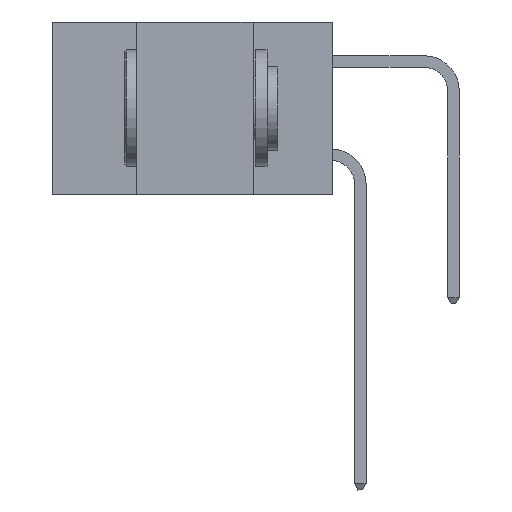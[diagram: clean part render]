
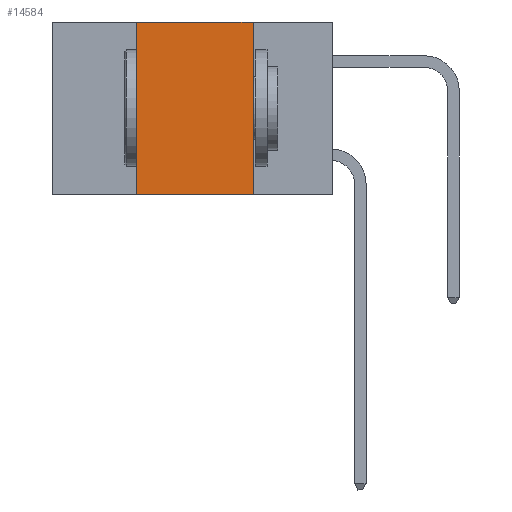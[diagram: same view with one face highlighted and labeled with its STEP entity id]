
A CAD part, left-side view. The second image highlights one B-rep face of the part: STEP entity #14584.
In plain terms, the highlighted planar face has unit normal (-1, 0, 0).
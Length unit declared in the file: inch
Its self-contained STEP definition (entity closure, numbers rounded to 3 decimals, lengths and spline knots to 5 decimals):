
#2361 = CARTESIAN_POINT ( 'NONE',  ( 0., 0.17, -0.37 ) ) ;
#2977 = CARTESIAN_POINT ( 'NONE',  ( 0., 0.6, 0. ) ) ;
#3004 = CARTESIAN_POINT ( 'NONE',  ( 0., 0.42, 0. ) ) ;
#4035 = CARTESIAN_POINT ( 'NONE',  ( 0., 0.42, -0.37 ) ) ;
#4650 = CARTESIAN_POINT ( 'NONE',  ( 0., 0.17, -0.37 ) ) ;
#4989 = AXIS2_PLACEMENT_3D ( 'NONE', #2977, #19009, #5336 ) ;
#5336 = DIRECTION ( 'NONE',  ( 0., 0., -1. ) ) ;
#6308 = VECTOR ( 'NONE', #9262, 39.37008 ) ;
#7500 = VERTEX_POINT ( 'NONE', #18423 ) ;
#7810 = VERTEX_POINT ( 'NONE', #23230 ) ;
#9262 = DIRECTION ( 'NONE',  ( 0., 0., -1. ) ) ;
#9483 = VECTOR ( 'NONE', #17723, 39.37008 ) ;
#10417 = CARTESIAN_POINT ( 'NONE',  ( 0., 0.6, -0.37 ) ) ;
#10583 = ORIENTED_EDGE ( 'NONE', *, *, #10824, .T. ) ;
#10824 = EDGE_CURVE ( 'NONE', #7810, #17937, #13853, .T. ) ;
#10895 = LINE ( 'NONE', #4035, #9483 ) ;
#12054 = VERTEX_POINT ( 'NONE', #3004 ) ;
#12106 = CARTESIAN_POINT ( 'NONE',  ( 0., 0.6, 0. ) ) ;
#12340 = EDGE_CURVE ( 'NONE', #7810, #12054, #10895, .T. ) ;
#13853 = LINE ( 'NONE', #10417, #19909 ) ;
#14584 = ADVANCED_FACE ( 'NONE', ( #21449 ), #25776, .F. ) ;
#15612 = LINE ( 'NONE', #12106, #21669 ) ;
#15916 = ORIENTED_EDGE ( 'NONE', *, *, #12340, .F. ) ;
#17723 = DIRECTION ( 'NONE',  ( 0., 0., 1. ) ) ;
#17937 = VERTEX_POINT ( 'NONE', #2361 ) ;
#18423 = CARTESIAN_POINT ( 'NONE',  ( 0., 0.17, 0. ) ) ;
#19009 = DIRECTION ( 'NONE',  ( 1., 0., 0. ) ) ;
#19909 = VECTOR ( 'NONE', #26361, 39.37008 ) ;
#19990 = EDGE_CURVE ( 'NONE', #12054, #7500, #15612, .T. ) ;
#20558 = ORIENTED_EDGE ( 'NONE', *, *, #21514, .F. ) ;
#21449 = FACE_OUTER_BOUND ( 'NONE', #25194, .T. ) ;
#21514 = EDGE_CURVE ( 'NONE', #7500, #17937, #29057, .T. ) ;
#21669 = VECTOR ( 'NONE', #28014, 39.37008 ) ;
#23230 = CARTESIAN_POINT ( 'NONE',  ( 0., 0.42, -0.37 ) ) ;
#25194 = EDGE_LOOP ( 'NONE', ( #20558, #26630, #15916, #10583 ) ) ;
#25776 = PLANE ( 'NONE',  #4989 ) ;
#26361 = DIRECTION ( 'NONE',  ( 0., -1., 0. ) ) ;
#26630 = ORIENTED_EDGE ( 'NONE', *, *, #19990, .F. ) ;
#28014 = DIRECTION ( 'NONE',  ( 0., -1., 0. ) ) ;
#29057 = LINE ( 'NONE', #4650, #6308 ) ;
